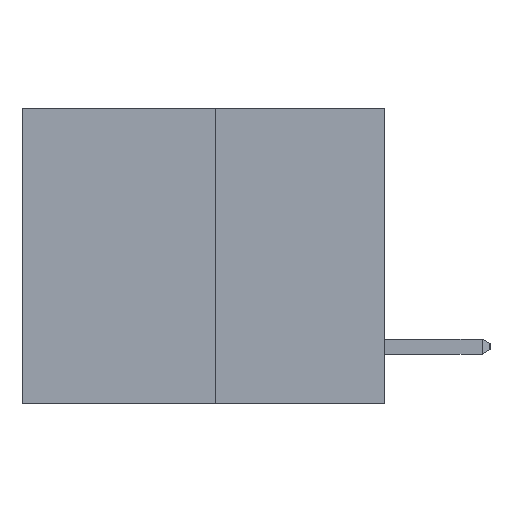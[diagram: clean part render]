
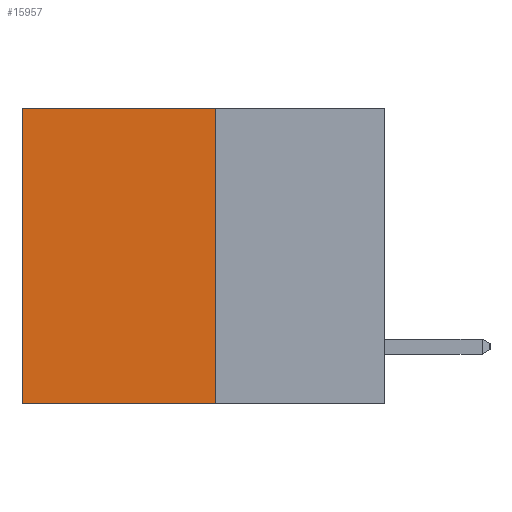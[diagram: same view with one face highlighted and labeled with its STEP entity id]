
A CAD part, left-side view. The second image highlights one B-rep face of the part: STEP entity #15957.
In plain terms, the highlighted planar face has unit normal (-1, 0, 0).
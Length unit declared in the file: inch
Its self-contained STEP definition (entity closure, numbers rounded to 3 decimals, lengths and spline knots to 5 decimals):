
#125 = ORIENTED_EDGE ( 'NONE', *, *, #15029, .T. ) ;
#524 = CARTESIAN_POINT ( 'NONE',  ( 0.3165, 0.28, 0. ) ) ;
#614 = VECTOR ( 'NONE', #7240, 39.37008 ) ;
#1056 = CARTESIAN_POINT ( 'NONE',  ( 0.3165, 0.28, -0.49 ) ) ;
#1251 = CARTESIAN_POINT ( 'NONE',  ( 0.3165, 0.6, -0.49 ) ) ;
#1429 = LINE ( 'NONE', #1251, #11543 ) ;
#1826 = EDGE_CURVE ( 'NONE', #10620, #13109, #6438, .T. ) ;
#3696 = CARTESIAN_POINT ( 'NONE',  ( 0.3165, 0.28, -0.49 ) ) ;
#4283 = DIRECTION ( 'NONE',  ( 1., 0., 0. ) ) ;
#4553 = PLANE ( 'NONE',  #17283 ) ;
#5910 = CARTESIAN_POINT ( 'NONE',  ( 0.3165, 0.28, -0.49 ) ) ;
#6202 = LINE ( 'NONE', #20875, #13556 ) ;
#6438 = LINE ( 'NONE', #12191, #614 ) ;
#7240 = DIRECTION ( 'NONE',  ( 0., 0., -1. ) ) ;
#7502 = ORIENTED_EDGE ( 'NONE', *, *, #17059, .F. ) ;
#9426 = DIRECTION ( 'NONE',  ( 0., 0., -1. ) ) ;
#10620 = VERTEX_POINT ( 'NONE', #524 ) ;
#11543 = VECTOR ( 'NONE', #14331, 39.37008 ) ;
#12191 = CARTESIAN_POINT ( 'NONE',  ( 0.3165, 0.28, -0.49 ) ) ;
#13109 = VERTEX_POINT ( 'NONE', #1056 ) ;
#13336 = VECTOR ( 'NONE', #18134, 39.37008 ) ;
#13556 = VECTOR ( 'NONE', #16256, 39.37008 ) ;
#14235 = EDGE_CURVE ( 'NONE', #16818, #16176, #1429, .T. ) ;
#14331 = DIRECTION ( 'NONE',  ( 0., 0., -1. ) ) ;
#14590 = ORIENTED_EDGE ( 'NONE', *, *, #14235, .T. ) ;
#15029 = EDGE_CURVE ( 'NONE', #10620, #16818, #6202, .T. ) ;
#15957 = ADVANCED_FACE ( 'NONE', ( #19398 ), #4553, .F. ) ;
#16176 = VERTEX_POINT ( 'NONE', #19223 ) ;
#16256 = DIRECTION ( 'NONE',  ( 0., 1., 0. ) ) ;
#16625 = CARTESIAN_POINT ( 'NONE',  ( 0.3165, 0.6, 0. ) ) ;
#16818 = VERTEX_POINT ( 'NONE', #16625 ) ;
#16829 = ORIENTED_EDGE ( 'NONE', *, *, #1826, .F. ) ;
#17059 = EDGE_CURVE ( 'NONE', #13109, #16176, #17604, .T. ) ;
#17283 = AXIS2_PLACEMENT_3D ( 'NONE', #5910, #4283, #9426 ) ;
#17604 = LINE ( 'NONE', #3696, #13336 ) ;
#18134 = DIRECTION ( 'NONE',  ( 0., 1., 0. ) ) ;
#19172 = EDGE_LOOP ( 'NONE', ( #14590, #7502, #16829, #125 ) ) ;
#19223 = CARTESIAN_POINT ( 'NONE',  ( 0.3165, 0.6, -0.49 ) ) ;
#19398 = FACE_OUTER_BOUND ( 'NONE', #19172, .T. ) ;
#20875 = CARTESIAN_POINT ( 'NONE',  ( 0.3165, 0.28, 0. ) ) ;
